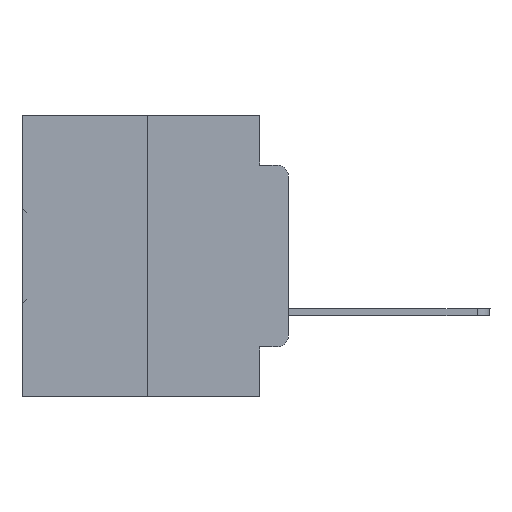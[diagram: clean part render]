
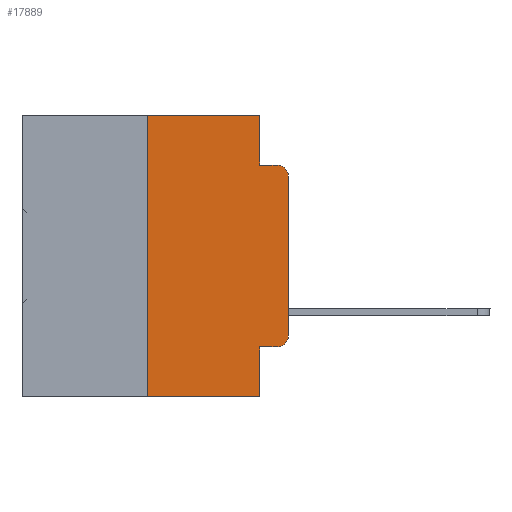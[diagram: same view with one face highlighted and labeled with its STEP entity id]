
A CAD part, left-side view. The second image highlights one B-rep face of the part: STEP entity #17889.
In plain terms, the highlighted planar face has unit normal (-1, 0, 0).
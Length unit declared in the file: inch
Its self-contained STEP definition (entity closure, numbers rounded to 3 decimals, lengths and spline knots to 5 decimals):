
#482 = ORIENTED_EDGE ( 'NONE', *, *, #31060, .F. ) ;
#563 = DIRECTION ( 'NONE',  ( 0., 0., -1. ) ) ;
#1255 = DIRECTION ( 'NONE',  ( -1., 0., 0. ) ) ;
#1567 = EDGE_CURVE ( 'NONE', #17657, #9312, #18247, .T. ) ;
#1950 = LINE ( 'NONE', #16714, #19293 ) ;
#3037 = EDGE_CURVE ( 'NONE', #27247, #17657, #17774, .T. ) ;
#3687 = CARTESIAN_POINT ( 'NONE',  ( 0., 0.02, -0.4115 ) ) ;
#4042 = DIRECTION ( 'NONE',  ( 0., -1., 0. ) ) ;
#4433 = EDGE_CURVE ( 'NONE', #18948, #16127, #14970, .T. ) ;
#4642 = CARTESIAN_POINT ( 'NONE',  ( 0., 0.473, 0. ) ) ;
#4787 = LINE ( 'NONE', #21467, #16934 ) ;
#5129 = EDGE_CURVE ( 'NONE', #9195, #16127, #4787, .T. ) ;
#5365 = CARTESIAN_POINT ( 'NONE',  ( 0., 0.051, 0. ) ) ;
#5893 = LINE ( 'NONE', #21306, #16450 ) ;
#5970 = EDGE_CURVE ( 'NONE', #29585, #11502, #1950, .T. ) ;
#5973 = FACE_OUTER_BOUND ( 'NONE', #18445, .T. ) ;
#6487 = DIRECTION ( 'NONE',  ( 0., -1., 0. ) ) ;
#6505 = ORIENTED_EDGE ( 'NONE', *, *, #5970, .T. ) ;
#7232 = DIRECTION ( 'NONE',  ( 0., 0., -1. ) ) ;
#7691 = EDGE_CURVE ( 'NONE', #11502, #24202, #32521, .T. ) ;
#8308 = VERTEX_POINT ( 'NONE', #24389 ) ;
#9064 = ORIENTED_EDGE ( 'NONE', *, *, #7691, .T. ) ;
#9195 = VERTEX_POINT ( 'NONE', #27871 ) ;
#9312 = VERTEX_POINT ( 'NONE', #16727 ) ;
#9709 = ORIENTED_EDGE ( 'NONE', *, *, #27179, .F. ) ;
#9898 = AXIS2_PLACEMENT_3D ( 'NONE', #15767, #10635, #28722 ) ;
#10151 = DIRECTION ( 'NONE',  ( 0., -1., 0. ) ) ;
#10350 = CARTESIAN_POINT ( 'NONE',  ( 0., 0.02, -0.0885 ) ) ;
#10635 = DIRECTION ( 'NONE',  ( 1., 0., 0. ) ) ;
#10780 = LINE ( 'NONE', #5365, #20558 ) ;
#11083 = AXIS2_PLACEMENT_3D ( 'NONE', #17875, #23141, #7232 ) ;
#11152 = ORIENTED_EDGE ( 'NONE', *, *, #18893, .T. ) ;
#11399 = CARTESIAN_POINT ( 'NONE',  ( 0., 0.02, -0.1085 ) ) ;
#11502 = VERTEX_POINT ( 'NONE', #3687 ) ;
#11965 = LINE ( 'NONE', #13482, #32981 ) ;
#12077 = CARTESIAN_POINT ( 'NONE',  ( 0., 0.25, 0. ) ) ;
#13482 = CARTESIAN_POINT ( 'NONE',  ( 0., 0.051, 0. ) ) ;
#13715 = ORIENTED_EDGE ( 'NONE', *, *, #5129, .F. ) ;
#13751 = CARTESIAN_POINT ( 'NONE',  ( 0., 0.25, 0. ) ) ;
#14033 = DIRECTION ( 'NONE',  ( 0., 0., -1. ) ) ;
#14970 = CIRCLE ( 'NONE', #28420, 0.02 ) ;
#15767 = CARTESIAN_POINT ( 'NONE',  ( 0., 0.473, 0. ) ) ;
#16127 = VERTEX_POINT ( 'NONE', #10350 ) ;
#16450 = VECTOR ( 'NONE', #26303, 39.37008 ) ;
#16714 = CARTESIAN_POINT ( 'NONE',  ( 0., 0.051, -0.4115 ) ) ;
#16727 = CARTESIAN_POINT ( 'NONE',  ( 0., 0.051, 0. ) ) ;
#16810 = DIRECTION ( 'NONE',  ( 0., 0., 1. ) ) ;
#16934 = VECTOR ( 'NONE', #6487, 39.37008 ) ;
#17145 = CARTESIAN_POINT ( 'NONE',  ( 0., 0., 0. ) ) ;
#17657 = VERTEX_POINT ( 'NONE', #13751 ) ;
#17774 = LINE ( 'NONE', #12077, #20549 ) ;
#17875 = CARTESIAN_POINT ( 'NONE',  ( 0., 0.02, -0.3915 ) ) ;
#17889 = ADVANCED_FACE ( 'NONE', ( #5973 ), #31208, .F. ) ;
#17901 = VECTOR ( 'NONE', #10151, 39.37008 ) ;
#18149 = LINE ( 'NONE', #17145, #18496 ) ;
#18190 = ORIENTED_EDGE ( 'NONE', *, *, #4433, .T. ) ;
#18247 = LINE ( 'NONE', #4642, #17901 ) ;
#18367 = DIRECTION ( 'NONE',  ( 0., 0., -1. ) ) ;
#18445 = EDGE_LOOP ( 'NONE', ( #32253, #18190, #13715, #9709, #30552, #19545, #11152, #482, #6505, #9064 ) ) ;
#18496 = VECTOR ( 'NONE', #16810, 39.37008 ) ;
#18893 = EDGE_CURVE ( 'NONE', #27247, #8308, #5893, .T. ) ;
#18948 = VERTEX_POINT ( 'NONE', #25293 ) ;
#19154 = CARTESIAN_POINT ( 'NONE',  ( 0., 0., -0.3915 ) ) ;
#19293 = VECTOR ( 'NONE', #4042, 39.37008 ) ;
#19430 = DIRECTION ( 'NONE',  ( 0., 0., 1. ) ) ;
#19545 = ORIENTED_EDGE ( 'NONE', *, *, #3037, .F. ) ;
#20278 = CARTESIAN_POINT ( 'NONE',  ( 0., 0.051, -0.4115 ) ) ;
#20549 = VECTOR ( 'NONE', #19430, 39.37008 ) ;
#20558 = VECTOR ( 'NONE', #563, 39.37008 ) ;
#21306 = CARTESIAN_POINT ( 'NONE',  ( 0., 0.473, -0.5 ) ) ;
#21467 = CARTESIAN_POINT ( 'NONE',  ( 0., 0.051, -0.0885 ) ) ;
#23141 = DIRECTION ( 'NONE',  ( -1., 0., 0. ) ) ;
#24202 = VERTEX_POINT ( 'NONE', #19154 ) ;
#24389 = CARTESIAN_POINT ( 'NONE',  ( 0., 0.051, -0.5 ) ) ;
#25293 = CARTESIAN_POINT ( 'NONE',  ( 0., 0., -0.1085 ) ) ;
#26303 = DIRECTION ( 'NONE',  ( 0., -1., 0. ) ) ;
#27179 = EDGE_CURVE ( 'NONE', #9312, #9195, #11965, .T. ) ;
#27247 = VERTEX_POINT ( 'NONE', #32110 ) ;
#27871 = CARTESIAN_POINT ( 'NONE',  ( 0., 0.051, -0.0885 ) ) ;
#28420 = AXIS2_PLACEMENT_3D ( 'NONE', #11399, #1255, #14033 ) ;
#28722 = DIRECTION ( 'NONE',  ( 0., 0., -1. ) ) ;
#29585 = VERTEX_POINT ( 'NONE', #20278 ) ;
#30552 = ORIENTED_EDGE ( 'NONE', *, *, #1567, .F. ) ;
#31060 = EDGE_CURVE ( 'NONE', #29585, #8308, #10780, .T. ) ;
#31206 = EDGE_CURVE ( 'NONE', #24202, #18948, #18149, .T. ) ;
#31208 = PLANE ( 'NONE',  #9898 ) ;
#32110 = CARTESIAN_POINT ( 'NONE',  ( 0., 0.25, -0.5 ) ) ;
#32253 = ORIENTED_EDGE ( 'NONE', *, *, #31206, .T. ) ;
#32521 = CIRCLE ( 'NONE', #11083, 0.02 ) ;
#32981 = VECTOR ( 'NONE', #18367, 39.37008 ) ;
